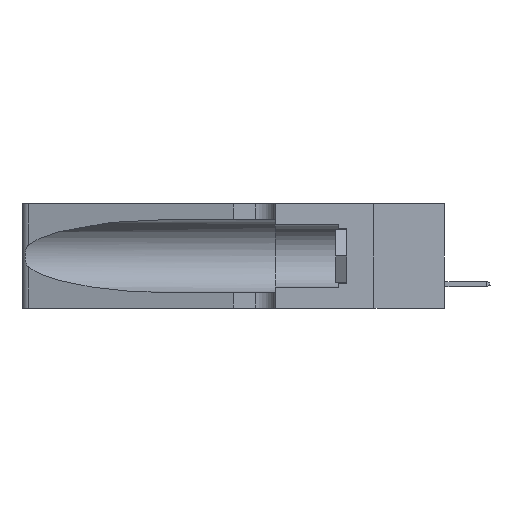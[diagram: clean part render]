
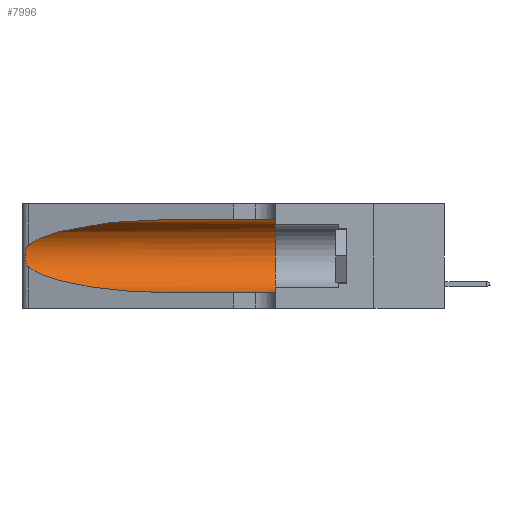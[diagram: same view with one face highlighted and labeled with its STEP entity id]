
A CAD part, left-side view. The second image highlights one B-rep face of the part: STEP entity #7996.
In plain terms, the highlighted cylindrical face has radius 3.308 mm (diameter 6.617 mm), a partial arc.
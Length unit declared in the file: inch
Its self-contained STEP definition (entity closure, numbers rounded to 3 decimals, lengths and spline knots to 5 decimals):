
#590 = EDGE_CURVE ( 'NONE', #11746, #12321, #16188, .T. ) ;
#1171 = CARTESIAN_POINT ( 'NONE',  ( 0.25487, 1.22718, 0.14631 ) ) ;
#1336 = ORIENTED_EDGE ( 'NONE', *, *, #2472, .T. ) ;
#1439 = CYLINDRICAL_SURFACE ( 'NONE', #11795, 0.13025 ) ;
#1468 = CARTESIAN_POINT ( 'NONE',  ( 0.1305, 0.35, 0.05475 ) ) ;
#2472 = EDGE_CURVE ( 'NONE', #9121, #11746, #16221, .T. ) ;
#2720 = VERTEX_POINT ( 'NONE', #13768 ) ;
#3359 = CARTESIAN_POINT ( 'NONE',  ( 0.25854, 1.2359, 0.20912 ) ) ;
#4380 = CARTESIAN_POINT ( 'NONE',  ( 0.1305, 0.35, 0.31525 ) ) ;
#4464 = VERTEX_POINT ( 'NONE', #4380 ) ;
#5440 = VECTOR ( 'NONE', #13185, 39.37008 ) ;
#5767 = DIRECTION ( 'NONE',  ( 0., 0., 1. ) ) ;
#5838 = ORIENTED_EDGE ( 'NONE', *, *, #590, .T. ) ;
#5946 = CARTESIAN_POINT ( 'NONE',  ( 0.25639, 1.23184, 0.21858 ) ) ;
#6084 = CARTESIAN_POINT ( 'NONE',  ( 0.25639, 1.23186, 0.15144 ) ) ;
#6744 = FACE_OUTER_BOUND ( 'NONE', #17473, .T. ) ;
#7090 = DIRECTION ( 'NONE',  ( 0., -1., 0. ) ) ;
#7217 = CARTESIAN_POINT ( 'NONE',  ( 0.25487, 1.22718, 0.22369 ) ) ;
#7293 = EDGE_CURVE ( 'NONE', #2720, #15928, #9682, .T. ) ;
#7996 = ADVANCED_FACE ( 'NONE', ( #6744 ), #1439, .F. ) ;
#8079 = CARTESIAN_POINT ( 'NONE',  ( 0.1305, 0.72297, 0.05475 ) ) ;
#8148 = CARTESIAN_POINT ( 'NONE',  ( 0.1305, 0.72297, 0.31525 ) ) ;
#9088 = CARTESIAN_POINT ( 'NONE',  ( 0.25487, 1.22718, 0.14631 ) ) ;
#9121 = VERTEX_POINT ( 'NONE', #11087 ) ;
#9145 = CARTESIAN_POINT ( 'NONE',  ( 0.25856, 1.23593, 0.16098 ) ) ;
#9192 = DIRECTION ( 'NONE',  ( 0., -1., 0. ) ) ;
#9395 = CARTESIAN_POINT ( 'NONE',  ( 0.1305, 1.61858, 0.185 ) ) ;
#9682 =( BOUNDED_CURVE ( )  B_SPLINE_CURVE ( 3, ( #8148, #18387, #9877, #12631 ),
 .UNSPECIFIED., .F., .T. ) 
 B_SPLINE_CURVE_WITH_KNOTS ( ( 4, 4 ),
 ( 1.5708, 2.84003 ),
 .UNSPECIFIED. ) 
 CURVE ( )  GEOMETRIC_REPRESENTATION_ITEM ( )  RATIONAL_B_SPLINE_CURVE ( ( 1., 0.87, 0.87, 1. ) ) 
 REPRESENTATION_ITEM ( '' )  );
#9877 = CARTESIAN_POINT ( 'NONE',  ( 0.2373, 1.15595, 0.28018 ) ) ;
#9928 = EDGE_CURVE ( 'NONE', #4464, #12321, #13542, .T. ) ;
#10007 = DIRECTION ( 'NONE',  ( 0., 1., 0. ) ) ;
#10703 = CARTESIAN_POINT ( 'NONE',  ( 0.25555, 1.22993, 0.14849 ) ) ;
#11087 = CARTESIAN_POINT ( 'NONE',  ( 0.25487, 1.22718, 0.14631 ) ) ;
#11450 = CARTESIAN_POINT ( 'NONE',  ( 0.1305, 1.61858, 0.31525 ) ) ;
#11585 = CARTESIAN_POINT ( 'NONE',  ( 0.1305, 0.35, 0.185 ) ) ;
#11657 = B_SPLINE_CURVE_WITH_KNOTS ( 'NONE', 3,
 ( #7217, #13064, #5946, #16175, #3359, #16362, #15101, #14831, #17969, #9145, #13620, #6084, #10703, #9088 ),
 .UNSPECIFIED., .F., .F.,
 ( 4, 2, 2, 2, 2, 2, 4 ),
 ( 0., 0.00027, 0.00053, 0.00107, 0.0016, 0.00187, 0.00214 ),
 .UNSPECIFIED. ) ;
#11746 = VERTEX_POINT ( 'NONE', #8079 ) ;
#11795 = AXIS2_PLACEMENT_3D ( 'NONE', #9395, #9192, #12131 ) ;
#12022 = ORIENTED_EDGE ( 'NONE', *, *, #18221, .F. ) ;
#12131 = DIRECTION ( 'NONE',  ( 0., 0., -1. ) ) ;
#12321 = VERTEX_POINT ( 'NONE', #1468 ) ;
#12631 = CARTESIAN_POINT ( 'NONE',  ( 0.25487, 1.22718, 0.22369 ) ) ;
#12975 = CARTESIAN_POINT ( 'NONE',  ( 0.2373, 1.15595, 0.08982 ) ) ;
#13064 = CARTESIAN_POINT ( 'NONE',  ( 0.25555, 1.22994, 0.2215 ) ) ;
#13168 = CARTESIAN_POINT ( 'NONE',  ( 0.18966, 0.96281, 0.05475 ) ) ;
#13185 = DIRECTION ( 'NONE',  ( 0., -1., 0. ) ) ;
#13542 = CIRCLE ( 'NONE', #16631, 0.13025 ) ;
#13620 = CARTESIAN_POINT ( 'NONE',  ( 0.25789, 1.23486, 0.15765 ) ) ;
#13768 = CARTESIAN_POINT ( 'NONE',  ( 0.1305, 0.72297, 0.31525 ) ) ;
#14423 = CARTESIAN_POINT ( 'NONE',  ( 0.1305, 0.72297, 0.05475 ) ) ;
#14504 = ORIENTED_EDGE ( 'NONE', *, *, #7293, .T. ) ;
#14831 = CARTESIAN_POINT ( 'NONE',  ( 0.26075, 1.23896, 0.178 ) ) ;
#15101 = CARTESIAN_POINT ( 'NONE',  ( 0.26075, 1.23896, 0.19203 ) ) ;
#15347 = ORIENTED_EDGE ( 'NONE', *, *, #18361, .T. ) ;
#15858 = CARTESIAN_POINT ( 'NONE',  ( 0.1305, 1.61858, 0.05475 ) ) ;
#15928 = VERTEX_POINT ( 'NONE', #17874 ) ;
#16175 = CARTESIAN_POINT ( 'NONE',  ( 0.25787, 1.23484, 0.2124 ) ) ;
#16188 = LINE ( 'NONE', #15858, #5440 ) ;
#16221 =( BOUNDED_CURVE ( )  B_SPLINE_CURVE ( 3, ( #1171, #12975, #13168, #14423 ),
 .UNSPECIFIED., .F., .F. ) 
 B_SPLINE_CURVE_WITH_KNOTS ( ( 4, 4 ),
 ( 3.44316, 4.71239 ),
 .UNSPECIFIED. ) 
 CURVE ( )  GEOMETRIC_REPRESENTATION_ITEM ( )  RATIONAL_B_SPLINE_CURVE ( ( 1., 0.87, 0.87, 1. ) ) 
 REPRESENTATION_ITEM ( '' )  );
#16362 = CARTESIAN_POINT ( 'NONE',  ( 0.26018, 1.23835, 0.19895 ) ) ;
#16405 = VECTOR ( 'NONE', #7090, 39.37008 ) ;
#16631 = AXIS2_PLACEMENT_3D ( 'NONE', #11585, #10007, #5767 ) ;
#17473 = EDGE_LOOP ( 'NONE', ( #14504, #15347, #1336, #5838, #18087, #12022 ) ) ;
#17874 = CARTESIAN_POINT ( 'NONE',  ( 0.25487, 1.22718, 0.22369 ) ) ;
#17969 = CARTESIAN_POINT ( 'NONE',  ( 0.26017, 1.23833, 0.17102 ) ) ;
#18087 = ORIENTED_EDGE ( 'NONE', *, *, #9928, .F. ) ;
#18221 = EDGE_CURVE ( 'NONE', #2720, #4464, #18965, .T. ) ;
#18361 = EDGE_CURVE ( 'NONE', #15928, #9121, #11657, .T. ) ;
#18387 = CARTESIAN_POINT ( 'NONE',  ( 0.18966, 0.96281, 0.31525 ) ) ;
#18965 = LINE ( 'NONE', #11450, #16405 ) ;
